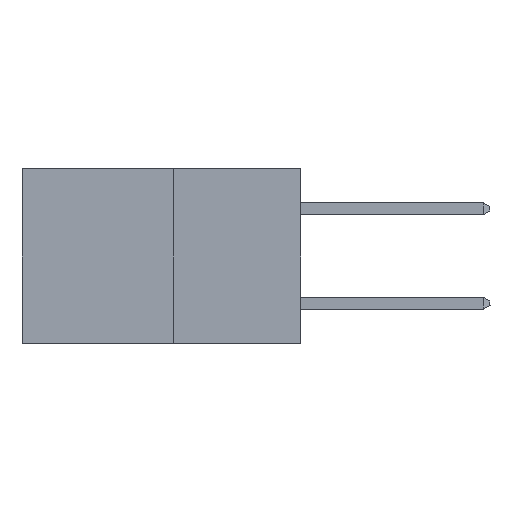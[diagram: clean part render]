
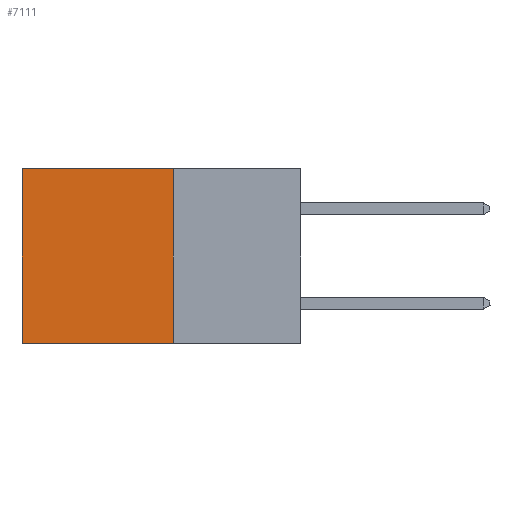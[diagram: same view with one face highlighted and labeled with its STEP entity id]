
A CAD part, left-side view. The second image highlights one B-rep face of the part: STEP entity #7111.
In plain terms, the highlighted planar face has unit normal (-1, 0, 0).
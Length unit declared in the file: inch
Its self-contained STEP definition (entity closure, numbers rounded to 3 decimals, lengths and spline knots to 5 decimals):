
#629 = VECTOR ( 'NONE', #26639, 39.37008 ) ;
#1285 = LINE ( 'NONE', #20360, #629 ) ;
#2396 = EDGE_LOOP ( 'NONE', ( #18853, #14688, #6178, #9514 ) ) ;
#3324 = VERTEX_POINT ( 'NONE', #14885 ) ;
#3476 = VERTEX_POINT ( 'NONE', #14490 ) ;
#4435 = DIRECTION ( 'NONE',  ( 1., 0., 0. ) ) ;
#4678 = EDGE_CURVE ( 'NONE', #20210, #18788, #8129, .T. ) ;
#6133 = AXIS2_PLACEMENT_3D ( 'NONE', #18904, #4435, #18996 ) ;
#6178 = ORIENTED_EDGE ( 'NONE', *, *, #10184, .F. ) ;
#7111 = ADVANCED_FACE ( 'NONE', ( #10971 ), #16958, .F. ) ;
#7883 = CARTESIAN_POINT ( 'NONE',  ( 0.277, 0.59, 0. ) ) ;
#8129 = LINE ( 'NONE', #17021, #23991 ) ;
#8894 = LINE ( 'NONE', #24631, #9562 ) ;
#9514 = ORIENTED_EDGE ( 'NONE', *, *, #4678, .T. ) ;
#9562 = VECTOR ( 'NONE', #12189, 39.37008 ) ;
#10184 = EDGE_CURVE ( 'NONE', #20210, #3324, #1285, .T. ) ;
#10338 = LINE ( 'NONE', #17029, #26155 ) ;
#10971 = FACE_OUTER_BOUND ( 'NONE', #2396, .T. ) ;
#12189 = DIRECTION ( 'NONE',  ( 0., 1., 0. ) ) ;
#14490 = CARTESIAN_POINT ( 'NONE',  ( 0.277, 0.59, -0.37 ) ) ;
#14688 = ORIENTED_EDGE ( 'NONE', *, *, #23770, .F. ) ;
#14885 = CARTESIAN_POINT ( 'NONE',  ( 0.277, 0.27, -0.37 ) ) ;
#16958 = PLANE ( 'NONE',  #6133 ) ;
#17021 = CARTESIAN_POINT ( 'NONE',  ( 0.277, 0.27, 0. ) ) ;
#17029 = CARTESIAN_POINT ( 'NONE',  ( 0.277, 0.59, -0.37 ) ) ;
#18788 = VERTEX_POINT ( 'NONE', #7883 ) ;
#18853 = ORIENTED_EDGE ( 'NONE', *, *, #21297, .T. ) ;
#18904 = CARTESIAN_POINT ( 'NONE',  ( 0.277, 0.27, -0.37 ) ) ;
#18996 = DIRECTION ( 'NONE',  ( 0., 0., -1. ) ) ;
#19072 = DIRECTION ( 'NONE',  ( 0., 0., -1. ) ) ;
#20210 = VERTEX_POINT ( 'NONE', #20248 ) ;
#20248 = CARTESIAN_POINT ( 'NONE',  ( 0.277, 0.27, 0. ) ) ;
#20360 = CARTESIAN_POINT ( 'NONE',  ( 0.277, 0.27, -0.37 ) ) ;
#21297 = EDGE_CURVE ( 'NONE', #18788, #3476, #10338, .T. ) ;
#23770 = EDGE_CURVE ( 'NONE', #3324, #3476, #8894, .T. ) ;
#23991 = VECTOR ( 'NONE', #25555, 39.37008 ) ;
#24631 = CARTESIAN_POINT ( 'NONE',  ( 0.277, 0.27, -0.37 ) ) ;
#25555 = DIRECTION ( 'NONE',  ( 0., 1., 0. ) ) ;
#26155 = VECTOR ( 'NONE', #19072, 39.37008 ) ;
#26639 = DIRECTION ( 'NONE',  ( 0., 0., -1. ) ) ;
